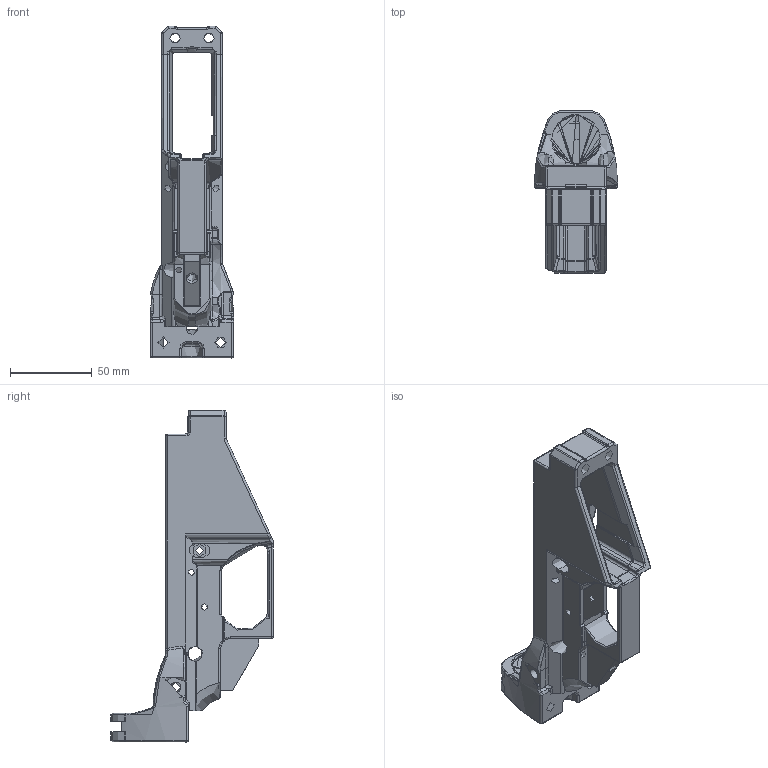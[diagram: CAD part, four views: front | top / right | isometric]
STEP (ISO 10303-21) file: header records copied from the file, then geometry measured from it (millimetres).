
FILE_DESCRIPTION(/* description */ (''),/* implementation_level */ '2;1');
FILE_NAME(/* name */ 'UBAR2 Forward Assist Low Shelf.stp',/* time_stamp */ '2022-02-28T22:52:41-06:00',/* author */ ('johne'),/* organization */ (''),/* preprocessor_version */ 'ST-DEVELOPER v18.1',/* originating_system */ 'Autodesk Inventor 2020',/* authorisation */ '');
FILE_SCHEMA (('AUTOMOTIVE_DESIGN { 1 0 10303 214 3 1 1 }'));
Products named in the file (1): UBAR Rev1 Forward Assist
Bounding box: 50.81 x 99.44 x 202.77 mm (x, y, z)
Volume: 156304.1 mm3; surface area: 58113.5 mm2
Topology: 1 solids, 1 shells, 942 faces, 2464 edges, 1468 vertices
Faces by surface type: cylinder 355, bspline 286, plane 147, torus 115, sphere 27, cone 12
Full cylindrical faces by diameter (mm): 3.81 x1, 3.969 x5, 5.182 x1, 5.334 x1, 6.35 x2, 6.477 x1, 6.604 x2, 6.858 x3, 7.938 x1, 9.55 x2
Entity records: 51180 total; most frequent: CARTESIAN_POINT 29540, ORIENTED_EDGE 4848, DIRECTION 4142, EDGE_CURVE 2424, AXIS2_PLACEMENT_3D 1687, VERTEX_POINT 1468, EDGE_LOOP 972, FACE_OUTER_BOUND 942
